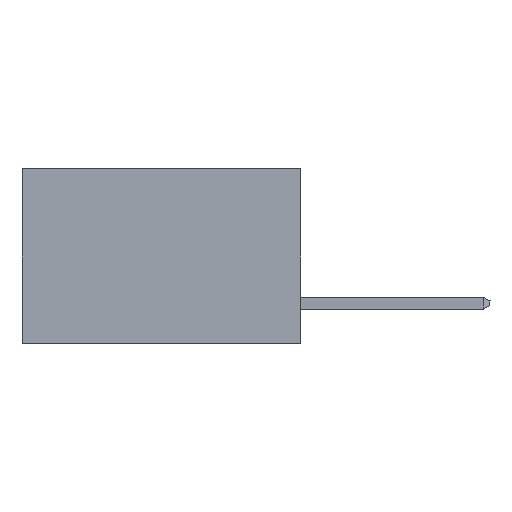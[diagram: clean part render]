
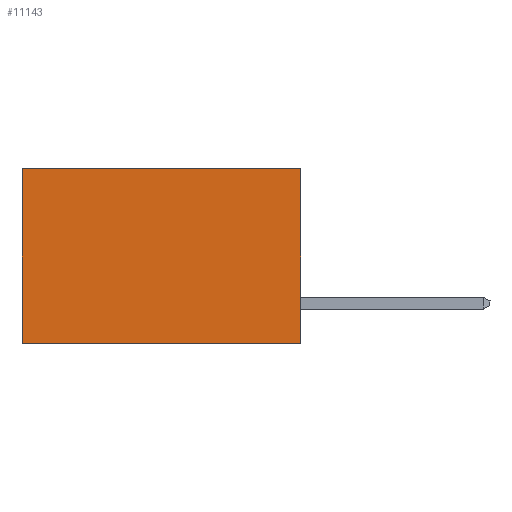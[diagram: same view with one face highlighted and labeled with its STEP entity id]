
A CAD part, left-side view. The second image highlights one B-rep face of the part: STEP entity #11143.
In plain terms, the highlighted planar face has unit normal (-1, 0, 0).
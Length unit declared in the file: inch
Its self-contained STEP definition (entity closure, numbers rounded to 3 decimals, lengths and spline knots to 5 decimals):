
#129 = VERTEX_POINT ( 'NONE', #14303 ) ;
#814 = CARTESIAN_POINT ( 'NONE',  ( 0.277, 0.59, -0.37 ) ) ;
#1300 = FACE_OUTER_BOUND ( 'NONE', #5961, .T. ) ;
#1460 = EDGE_CURVE ( 'NONE', #11933, #16284, #7126, .T. ) ;
#1785 = ORIENTED_EDGE ( 'NONE', *, *, #3587, .T. ) ;
#1964 = CARTESIAN_POINT ( 'NONE',  ( 0.277, 0., -0.37 ) ) ;
#3221 = DIRECTION ( 'NONE',  ( 0., 1., 0. ) ) ;
#3239 = LINE ( 'NONE', #814, #5992 ) ;
#3587 = EDGE_CURVE ( 'NONE', #15707, #129, #3239, .T. ) ;
#3677 = ORIENTED_EDGE ( 'NONE', *, *, #1460, .F. ) ;
#4173 = DIRECTION ( 'NONE',  ( 0., 0., -1. ) ) ;
#4968 = ORIENTED_EDGE ( 'NONE', *, *, #5039, .T. ) ;
#5039 = EDGE_CURVE ( 'NONE', #11933, #15707, #14621, .T. ) ;
#5905 = DIRECTION ( 'NONE',  ( 0., 0., -1. ) ) ;
#5961 = EDGE_LOOP ( 'NONE', ( #1785, #8944, #3677, #4968 ) ) ;
#5992 = VECTOR ( 'NONE', #14065, 39.37008 ) ;
#6271 = CARTESIAN_POINT ( 'NONE',  ( 0.277, 0., -0.37 ) ) ;
#6824 = CARTESIAN_POINT ( 'NONE',  ( 0.277, 0., -0.37 ) ) ;
#7003 = LINE ( 'NONE', #12536, #17003 ) ;
#7126 = LINE ( 'NONE', #6271, #10670 ) ;
#8944 = ORIENTED_EDGE ( 'NONE', *, *, #9743, .F. ) ;
#9743 = EDGE_CURVE ( 'NONE', #16284, #129, #7003, .T. ) ;
#10670 = VECTOR ( 'NONE', #5905, 39.37008 ) ;
#10839 = PLANE ( 'NONE',  #14203 ) ;
#11015 = CARTESIAN_POINT ( 'NONE',  ( 0.277, 0., 0. ) ) ;
#11110 = CARTESIAN_POINT ( 'NONE',  ( 0.277, 0., 0. ) ) ;
#11143 = ADVANCED_FACE ( 'NONE', ( #1300 ), #10839, .F. ) ;
#11159 = VECTOR ( 'NONE', #3221, 39.37008 ) ;
#11299 = DIRECTION ( 'NONE',  ( 0., 1., 0. ) ) ;
#11933 = VERTEX_POINT ( 'NONE', #11110 ) ;
#12139 = DIRECTION ( 'NONE',  ( 1., 0., 0. ) ) ;
#12536 = CARTESIAN_POINT ( 'NONE',  ( 0.277, 0., -0.37 ) ) ;
#12691 = CARTESIAN_POINT ( 'NONE',  ( 0.277, 0.59, 0. ) ) ;
#14065 = DIRECTION ( 'NONE',  ( 0., 0., -1. ) ) ;
#14203 = AXIS2_PLACEMENT_3D ( 'NONE', #6824, #12139, #4173 ) ;
#14303 = CARTESIAN_POINT ( 'NONE',  ( 0.277, 0.59, -0.37 ) ) ;
#14621 = LINE ( 'NONE', #11015, #11159 ) ;
#15707 = VERTEX_POINT ( 'NONE', #12691 ) ;
#16284 = VERTEX_POINT ( 'NONE', #1964 ) ;
#17003 = VECTOR ( 'NONE', #11299, 39.37008 ) ;
